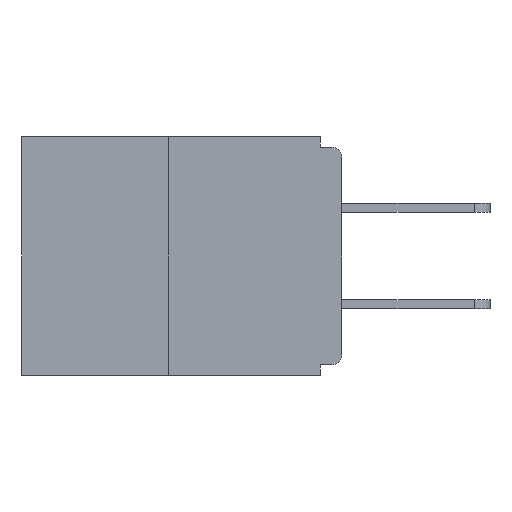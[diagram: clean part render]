
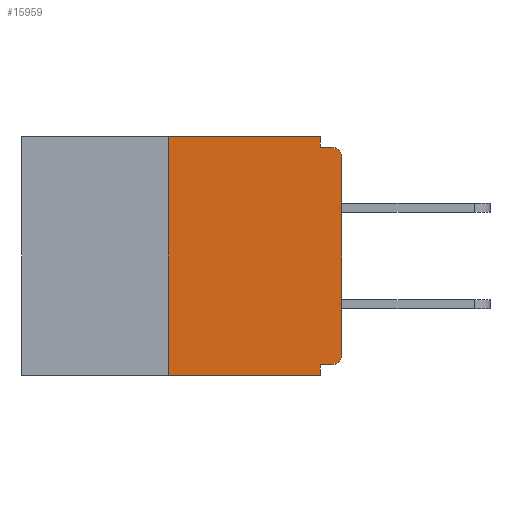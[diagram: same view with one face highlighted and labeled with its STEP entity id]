
A CAD part, left-side view. The second image highlights one B-rep face of the part: STEP entity #15959.
In plain terms, the highlighted planar face has unit normal (-1, 0, 0).
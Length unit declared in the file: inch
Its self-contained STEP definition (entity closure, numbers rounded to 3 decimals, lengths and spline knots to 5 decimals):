
#189 = ORIENTED_EDGE ( 'NONE', *, *, #6925, .T. ) ;
#644 = ORIENTED_EDGE ( 'NONE', *, *, #9830, .T. ) ;
#687 = VERTEX_POINT ( 'NONE', #13260 ) ;
#1014 = AXIS2_PLACEMENT_3D ( 'NONE', #5578, #17707, #11684 ) ;
#1219 = ORIENTED_EDGE ( 'NONE', *, *, #15649, .F. ) ;
#1533 = CARTESIAN_POINT ( 'NONE',  ( 0., 0., 0. ) ) ;
#2460 = AXIS2_PLACEMENT_3D ( 'NONE', #10209, #10347, #17985 ) ;
#2555 = PLANE ( 'NONE',  #2460 ) ;
#2668 = CARTESIAN_POINT ( 'NONE',  ( 0., 0.031, 0. ) ) ;
#2802 = DIRECTION ( 'NONE',  ( 0., 0., -1. ) ) ;
#3061 = DIRECTION ( 'NONE',  ( 0., 0., 1. ) ) ;
#3410 = DIRECTION ( 'NONE',  ( 0., -1., 0. ) ) ;
#3532 = CARTESIAN_POINT ( 'NONE',  ( 0., 0.46, 0. ) ) ;
#3928 = CARTESIAN_POINT ( 'NONE',  ( 0., 0.46, -0.343 ) ) ;
#4003 = VERTEX_POINT ( 'NONE', #13189 ) ;
#4093 = CIRCLE ( 'NONE', #1014, 0.015 ) ;
#4210 = CARTESIAN_POINT ( 'NONE',  ( 0., 0., -0.03 ) ) ;
#4507 = VECTOR ( 'NONE', #3061, 39.37008 ) ;
#4572 = VECTOR ( 'NONE', #8261, 39.37008 ) ;
#4796 = CARTESIAN_POINT ( 'NONE',  ( 0., 0.031, -0.328 ) ) ;
#5014 = ORIENTED_EDGE ( 'NONE', *, *, #14330, .F. ) ;
#5109 = VECTOR ( 'NONE', #7508, 39.37008 ) ;
#5181 = CARTESIAN_POINT ( 'NONE',  ( 0., 0.031, 0. ) ) ;
#5307 = VERTEX_POINT ( 'NONE', #15211 ) ;
#5578 = CARTESIAN_POINT ( 'NONE',  ( 0., 0.015, -0.03 ) ) ;
#5979 = VERTEX_POINT ( 'NONE', #6696 ) ;
#6359 = VERTEX_POINT ( 'NONE', #9261 ) ;
#6369 = VECTOR ( 'NONE', #3410, 39.37008 ) ;
#6696 = CARTESIAN_POINT ( 'NONE',  ( 0., 0.015, -0.328 ) ) ;
#6925 = EDGE_CURVE ( 'NONE', #4003, #12290, #16675, .T. ) ;
#6931 = ORIENTED_EDGE ( 'NONE', *, *, #8318, .T. ) ;
#6943 = CARTESIAN_POINT ( 'NONE',  ( 0., 0.015, -0.313 ) ) ;
#7138 = LINE ( 'NONE', #2668, #8552 ) ;
#7193 = CARTESIAN_POINT ( 'NONE',  ( 0., 0.25, 0. ) ) ;
#7206 = DIRECTION ( 'NONE',  ( -1., 0., 0. ) ) ;
#7508 = DIRECTION ( 'NONE',  ( 0., 1., 0. ) ) ;
#7814 = EDGE_LOOP ( 'NONE', ( #12679, #14542, #189, #9490, #9527, #6931, #644, #13547, #1219, #5014 ) ) ;
#8031 = LINE ( 'NONE', #7193, #11629 ) ;
#8261 = DIRECTION ( 'NONE',  ( 0., -1., 0. ) ) ;
#8318 = EDGE_CURVE ( 'NONE', #5979, #687, #9984, .T. ) ;
#8525 = DIRECTION ( 'NONE',  ( 0., 0., -1. ) ) ;
#8552 = VECTOR ( 'NONE', #2802, 39.37008 ) ;
#9221 = VERTEX_POINT ( 'NONE', #5181 ) ;
#9261 = CARTESIAN_POINT ( 'NONE',  ( 0., 0.015, -0.015 ) ) ;
#9490 = ORIENTED_EDGE ( 'NONE', *, *, #11896, .F. ) ;
#9527 = ORIENTED_EDGE ( 'NONE', *, *, #12054, .F. ) ;
#9809 = VECTOR ( 'NONE', #11643, 39.37008 ) ;
#9830 = EDGE_CURVE ( 'NONE', #687, #17605, #18260, .T. ) ;
#9984 = CIRCLE ( 'NONE', #19142, 0.015 ) ;
#10209 = CARTESIAN_POINT ( 'NONE',  ( 0., 0.46, 0. ) ) ;
#10347 = DIRECTION ( 'NONE',  ( 1., 0., 0. ) ) ;
#10396 = LINE ( 'NONE', #17336, #6369 ) ;
#11629 = VECTOR ( 'NONE', #14697, 39.37008 ) ;
#11643 = DIRECTION ( 'NONE',  ( 0., 0., -1. ) ) ;
#11684 = DIRECTION ( 'NONE',  ( 0., 0., -1. ) ) ;
#11896 = EDGE_CURVE ( 'NONE', #12088, #12290, #17902, .T. ) ;
#12054 = EDGE_CURVE ( 'NONE', #5979, #12088, #15299, .T. ) ;
#12088 = VERTEX_POINT ( 'NONE', #4796 ) ;
#12290 = VERTEX_POINT ( 'NONE', #17331 ) ;
#12679 = ORIENTED_EDGE ( 'NONE', *, *, #14856, .F. ) ;
#13189 = CARTESIAN_POINT ( 'NONE',  ( 0., 0.25, -0.343 ) ) ;
#13260 = CARTESIAN_POINT ( 'NONE',  ( 0., 0., -0.313 ) ) ;
#13540 = VECTOR ( 'NONE', #15735, 39.37008 ) ;
#13547 = ORIENTED_EDGE ( 'NONE', *, *, #14413, .T. ) ;
#14330 = EDGE_CURVE ( 'NONE', #9221, #5307, #7138, .T. ) ;
#14413 = EDGE_CURVE ( 'NONE', #17605, #6359, #4093, .T. ) ;
#14542 = ORIENTED_EDGE ( 'NONE', *, *, #15183, .F. ) ;
#14697 = DIRECTION ( 'NONE',  ( 0., 0., 1. ) ) ;
#14856 = EDGE_CURVE ( 'NONE', #19192, #9221, #16863, .T. ) ;
#15183 = EDGE_CURVE ( 'NONE', #4003, #19192, #8031, .T. ) ;
#15211 = CARTESIAN_POINT ( 'NONE',  ( 0., 0.031, -0.015 ) ) ;
#15299 = LINE ( 'NONE', #18131, #5109 ) ;
#15649 = EDGE_CURVE ( 'NONE', #5307, #6359, #10396, .T. ) ;
#15735 = DIRECTION ( 'NONE',  ( 0., -1., 0. ) ) ;
#15959 = ADVANCED_FACE ( 'NONE', ( #17530 ), #2555, .F. ) ;
#16675 = LINE ( 'NONE', #3928, #4572 ) ;
#16863 = LINE ( 'NONE', #3532, #13540 ) ;
#17331 = CARTESIAN_POINT ( 'NONE',  ( 0., 0.031, -0.343 ) ) ;
#17336 = CARTESIAN_POINT ( 'NONE',  ( 0., 0., -0.015 ) ) ;
#17530 = FACE_OUTER_BOUND ( 'NONE', #7814, .T. ) ;
#17605 = VERTEX_POINT ( 'NONE', #4210 ) ;
#17707 = DIRECTION ( 'NONE',  ( -1., 0., 0. ) ) ;
#17795 = CARTESIAN_POINT ( 'NONE',  ( 0., 0.031, -0.343 ) ) ;
#17902 = LINE ( 'NONE', #17795, #9809 ) ;
#17985 = DIRECTION ( 'NONE',  ( 0., 0., -1. ) ) ;
#18131 = CARTESIAN_POINT ( 'NONE',  ( 0., 0., -0.328 ) ) ;
#18260 = LINE ( 'NONE', #1533, #4507 ) ;
#18402 = CARTESIAN_POINT ( 'NONE',  ( 0., 0.25, 0. ) ) ;
#19142 = AXIS2_PLACEMENT_3D ( 'NONE', #6943, #7206, #8525 ) ;
#19192 = VERTEX_POINT ( 'NONE', #18402 ) ;
